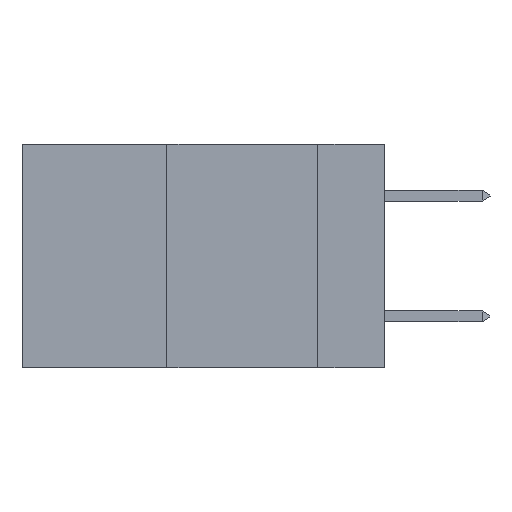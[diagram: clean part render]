
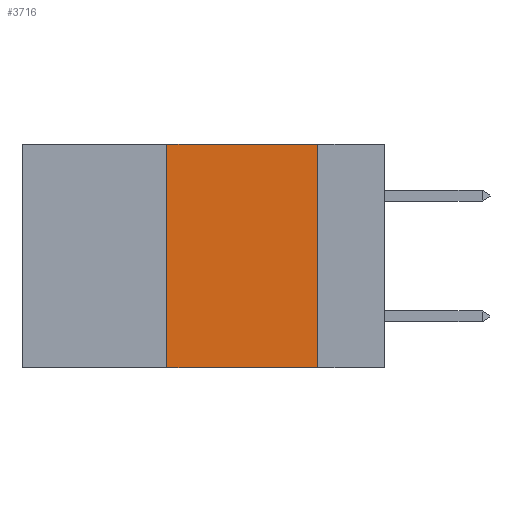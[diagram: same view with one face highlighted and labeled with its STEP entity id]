
A CAD part, left-side view. The second image highlights one B-rep face of the part: STEP entity #3716.
In plain terms, the highlighted planar face has unit normal (-1, 0, 0).
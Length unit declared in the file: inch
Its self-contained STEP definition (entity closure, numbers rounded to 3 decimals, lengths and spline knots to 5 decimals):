
#1540 = DIRECTION ( 'NONE',  ( 0., -1., 0. ) ) ;
#2015 = VERTEX_POINT ( 'NONE', #11929 ) ;
#3263 = CARTESIAN_POINT ( 'NONE',  ( 0., 0.11, 0. ) ) ;
#3716 = ADVANCED_FACE ( 'NONE', ( #24694 ), #10120, .F. ) ;
#5260 = VECTOR ( 'NONE', #1540, 39.37008 ) ;
#5503 = VERTEX_POINT ( 'NONE', #3263 ) ;
#5838 = LINE ( 'NONE', #18052, #21880 ) ;
#7489 = DIRECTION ( 'NONE',  ( 0., -1., 0. ) ) ;
#7723 = ORIENTED_EDGE ( 'NONE', *, *, #20283, .F. ) ;
#7738 = LINE ( 'NONE', #20392, #5260 ) ;
#7900 = ORIENTED_EDGE ( 'NONE', *, *, #10247, .F. ) ;
#9469 = LINE ( 'NONE', #20054, #18983 ) ;
#9673 = EDGE_LOOP ( 'NONE', ( #7900, #23259, #7723, #25313 ) ) ;
#10120 = PLANE ( 'NONE',  #13200 ) ;
#10247 = EDGE_CURVE ( 'NONE', #5503, #2015, #5838, .T. ) ;
#11929 = CARTESIAN_POINT ( 'NONE',  ( 0., 0.11, -0.37 ) ) ;
#12043 = DIRECTION ( 'NONE',  ( 1., 0., 0. ) ) ;
#12072 = EDGE_CURVE ( 'NONE', #16298, #2015, #7738, .T. ) ;
#13200 = AXIS2_PLACEMENT_3D ( 'NONE', #14220, #12043, #20583 ) ;
#13570 = DIRECTION ( 'NONE',  ( 0., 0., 1. ) ) ;
#14220 = CARTESIAN_POINT ( 'NONE',  ( 0., 0.6, 0. ) ) ;
#16029 = VECTOR ( 'NONE', #7489, 39.37008 ) ;
#16298 = VERTEX_POINT ( 'NONE', #22363 ) ;
#18052 = CARTESIAN_POINT ( 'NONE',  ( 0., 0.11, 0. ) ) ;
#18983 = VECTOR ( 'NONE', #13570, 39.37008 ) ;
#20054 = CARTESIAN_POINT ( 'NONE',  ( 0., 0.36, 0. ) ) ;
#20283 = EDGE_CURVE ( 'NONE', #16298, #23329, #9469, .T. ) ;
#20392 = CARTESIAN_POINT ( 'NONE',  ( 0., 0.6, -0.37 ) ) ;
#20583 = DIRECTION ( 'NONE',  ( 0., 0., -1. ) ) ;
#20891 = CARTESIAN_POINT ( 'NONE',  ( 0., 0.36, 0. ) ) ;
#21880 = VECTOR ( 'NONE', #22720, 39.37008 ) ;
#22363 = CARTESIAN_POINT ( 'NONE',  ( 0., 0.36, -0.37 ) ) ;
#22720 = DIRECTION ( 'NONE',  ( 0., 0., -1. ) ) ;
#23259 = ORIENTED_EDGE ( 'NONE', *, *, #25884, .F. ) ;
#23329 = VERTEX_POINT ( 'NONE', #20891 ) ;
#24694 = FACE_OUTER_BOUND ( 'NONE', #9673, .T. ) ;
#24776 = LINE ( 'NONE', #26295, #16029 ) ;
#25313 = ORIENTED_EDGE ( 'NONE', *, *, #12072, .T. ) ;
#25884 = EDGE_CURVE ( 'NONE', #23329, #5503, #24776, .T. ) ;
#26295 = CARTESIAN_POINT ( 'NONE',  ( 0., 0.6, 0. ) ) ;
